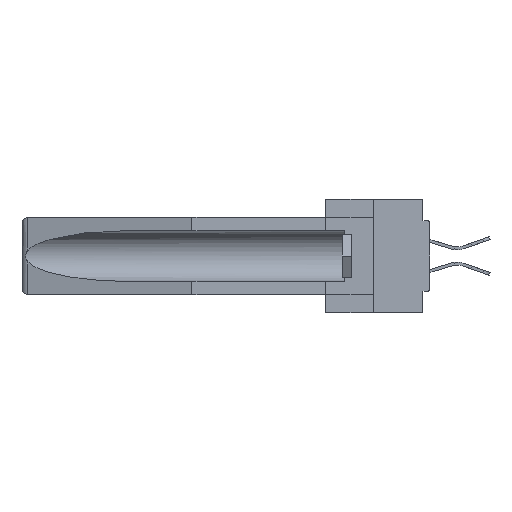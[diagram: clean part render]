
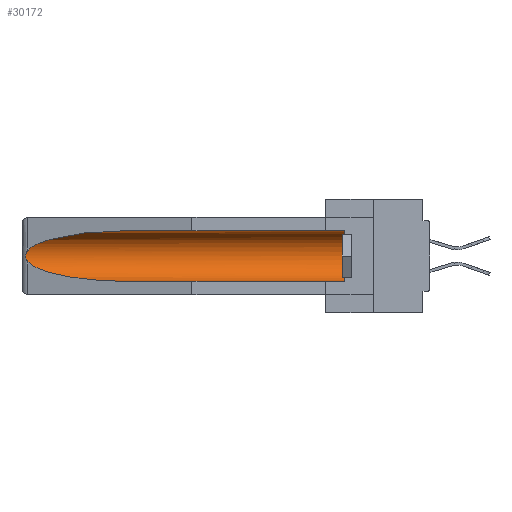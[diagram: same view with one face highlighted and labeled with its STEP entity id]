
A CAD part, left-side view. The second image highlights one B-rep face of the part: STEP entity #30172.
In plain terms, the highlighted cylindrical face has radius 2.857 mm (diameter 5.715 mm), a partial arc.
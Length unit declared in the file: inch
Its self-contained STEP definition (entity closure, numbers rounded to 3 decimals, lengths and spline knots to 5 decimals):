
#164 = CARTESIAN_POINT ( 'NONE',  ( 0.26537, 1.52718, -0.19328 ) ) ;
#1880 = CIRCLE ( 'NONE', #13676, 0.1125 ) ;
#4442 = EDGE_CURVE ( 'NONE', #10927, #16342, #15980, .T. ) ;
#5326 = CARTESIAN_POINT ( 'NONE',  ( 0.26537, 1.52718, -0.14972 ) ) ;
#6687 = CARTESIAN_POINT ( 'NONE',  ( 0.26654, 1.53092, -0.15636 ) ) ;
#7798 = VECTOR ( 'NONE', #37877, 39.37008 ) ;
#7871 = CARTESIAN_POINT ( 'NONE',  ( 0.155, 1.07973, -0.059 ) ) ;
#8500 = DIRECTION ( 'NONE',  ( 0., 1., 0. ) ) ;
#8683 = ORIENTED_EDGE ( 'NONE', *, *, #11559, .T. ) ;
#10927 = VERTEX_POINT ( 'NONE', #19259 ) ;
#11559 = EDGE_CURVE ( 'NONE', #22533, #16336, #12990, .T. ) ;
#12375 = ORIENTED_EDGE ( 'NONE', *, *, #24691, .T. ) ;
#12990 =( BOUNDED_CURVE ( )  B_SPLINE_CURVE ( 3, ( #20230, #32289, #14204, #38350 ),
 .UNSPECIFIED., .F., .F. ) 
 B_SPLINE_CURVE_WITH_KNOTS ( ( 4, 4 ),
 ( 4.71239, 6.08839 ),
 .UNSPECIFIED. ) 
 CURVE ( )  GEOMETRIC_REPRESENTATION_ITEM ( )  RATIONAL_B_SPLINE_CURVE ( ( 1., 0.848, 0.848, 1. ) ) 
 REPRESENTATION_ITEM ( '' )  );
#13128 = VERTEX_POINT ( 'NONE', #30870 ) ;
#13162 = AXIS2_PLACEMENT_3D ( 'NONE', #26617, #8500, #29916 ) ;
#13676 = AXIS2_PLACEMENT_3D ( 'NONE', #35929, #33210, #36054 ) ;
#14204 = CARTESIAN_POINT ( 'NONE',  ( 0.25451, 1.48313, -0.09465 ) ) ;
#15980 = LINE ( 'NONE', #25186, #7798 ) ;
#16218 = ORIENTED_EDGE ( 'NONE', *, *, #31142, .T. ) ;
#16336 = VERTEX_POINT ( 'NONE', #35671 ) ;
#16342 = VERTEX_POINT ( 'NONE', #20113 ) ;
#17357 = ORIENTED_EDGE ( 'NONE', *, *, #4442, .F. ) ;
#17467 = CARTESIAN_POINT ( 'NONE',  ( 0.25451, 1.48313, -0.24835 ) ) ;
#18372 = EDGE_CURVE ( 'NONE', #13128, #22533, #19499, .T. ) ;
#19135 = CARTESIAN_POINT ( 'NONE',  ( 0.2673, 1.5327, -0.16383 ) ) ;
#19259 = CARTESIAN_POINT ( 'NONE',  ( 0.155, 0.126, -0.284 ) ) ;
#19352 =( BOUNDED_CURVE ( )  B_SPLINE_CURVE ( 3, ( #20772, #17467, #39013, #23753 ),
 .UNSPECIFIED., .F., .F. ) 
 B_SPLINE_CURVE_WITH_KNOTS ( ( 4, 4 ),
 ( 0.1948, 1.5708 ),
 .UNSPECIFIED. ) 
 CURVE ( )  GEOMETRIC_REPRESENTATION_ITEM ( )  RATIONAL_B_SPLINE_CURVE ( ( 1., 0.848, 0.848, 1. ) ) 
 REPRESENTATION_ITEM ( '' )  );
#19499 = LINE ( 'NONE', #37167, #24796 ) ;
#20113 = CARTESIAN_POINT ( 'NONE',  ( 0.155, 1.07973, -0.284 ) ) ;
#20230 = CARTESIAN_POINT ( 'NONE',  ( 0.155, 1.07973, -0.059 ) ) ;
#20438 = FACE_OUTER_BOUND ( 'NONE', #39871, .T. ) ;
#20772 = CARTESIAN_POINT ( 'NONE',  ( 0.26537, 1.52718, -0.19328 ) ) ;
#20946 = VERTEX_POINT ( 'NONE', #164 ) ;
#22482 = CARTESIAN_POINT ( 'NONE',  ( 0.2675, 1.53308, -0.17534 ) ) ;
#22533 = VERTEX_POINT ( 'NONE', #7871 ) ;
#23753 = CARTESIAN_POINT ( 'NONE',  ( 0.155, 1.07973, -0.284 ) ) ;
#24691 = EDGE_CURVE ( 'NONE', #16336, #20946, #32463, .T. ) ;
#24796 = VECTOR ( 'NONE', #30838, 39.37008 ) ;
#25048 = CARTESIAN_POINT ( 'NONE',  ( 0.26597, 1.52961, -0.15275 ) ) ;
#25186 = CARTESIAN_POINT ( 'NONE',  ( 0.155, -0.30754, -0.284 ) ) ;
#25320 = CARTESIAN_POINT ( 'NONE',  ( 0.26597, 1.5296, -0.19026 ) ) ;
#26028 = EDGE_CURVE ( 'NONE', #20946, #16342, #19352, .T. ) ;
#26617 = CARTESIAN_POINT ( 'NONE',  ( 0.155, -0.30754, -0.1715 ) ) ;
#28171 = CARTESIAN_POINT ( 'NONE',  ( 0.26655, 1.53094, -0.18657 ) ) ;
#29916 = DIRECTION ( 'NONE',  ( 0., 0., 1. ) ) ;
#30172 = ADVANCED_FACE ( 'NONE', ( #20438 ), #32088, .F. ) ;
#30838 = DIRECTION ( 'NONE',  ( 0., 1., 0. ) ) ;
#30870 = CARTESIAN_POINT ( 'NONE',  ( 0.155, 0.126, -0.059 ) ) ;
#31142 = EDGE_CURVE ( 'NONE', #10927, #13128, #1880, .T. ) ;
#31698 = CARTESIAN_POINT ( 'NONE',  ( 0.26537, 1.52718, -0.19328 ) ) ;
#32088 = CYLINDRICAL_SURFACE ( 'NONE', #13162, 0.1125 ) ;
#32289 = CARTESIAN_POINT ( 'NONE',  ( 0.21114, 1.30732, -0.059 ) ) ;
#32421 = ORIENTED_EDGE ( 'NONE', *, *, #26028, .T. ) ;
#32463 = B_SPLINE_CURVE_WITH_KNOTS ( 'NONE', 3,
 ( #5326, #25048, #6687, #19135, #37621, #22482, #34236, #28171, #25320, #31698 ),
 .UNSPECIFIED., .F., .F.,
 ( 4, 2, 2, 2, 4 ),
 ( 0., 0.00029, 0.00058, 0.00087, 0.00117 ),
 .UNSPECIFIED. ) ;
#33210 = DIRECTION ( 'NONE',  ( 0., -1., 0. ) ) ;
#34236 = CARTESIAN_POINT ( 'NONE',  ( 0.2673, 1.53269, -0.17917 ) ) ;
#35671 = CARTESIAN_POINT ( 'NONE',  ( 0.26537, 1.52718, -0.14972 ) ) ;
#35929 = CARTESIAN_POINT ( 'NONE',  ( 0.155, 0.126, -0.1715 ) ) ;
#36054 = DIRECTION ( 'NONE',  ( 0., 0., 1. ) ) ;
#36799 = ORIENTED_EDGE ( 'NONE', *, *, #18372, .T. ) ;
#37167 = CARTESIAN_POINT ( 'NONE',  ( 0.155, -0.30754, -0.059 ) ) ;
#37621 = CARTESIAN_POINT ( 'NONE',  ( 0.2675, 1.53308, -0.16763 ) ) ;
#37877 = DIRECTION ( 'NONE',  ( 0., 1., 0. ) ) ;
#38350 = CARTESIAN_POINT ( 'NONE',  ( 0.26537, 1.52718, -0.14972 ) ) ;
#39013 = CARTESIAN_POINT ( 'NONE',  ( 0.21114, 1.30732, -0.284 ) ) ;
#39871 = EDGE_LOOP ( 'NONE', ( #8683, #12375, #32421, #17357, #16218, #36799 ) ) ;
